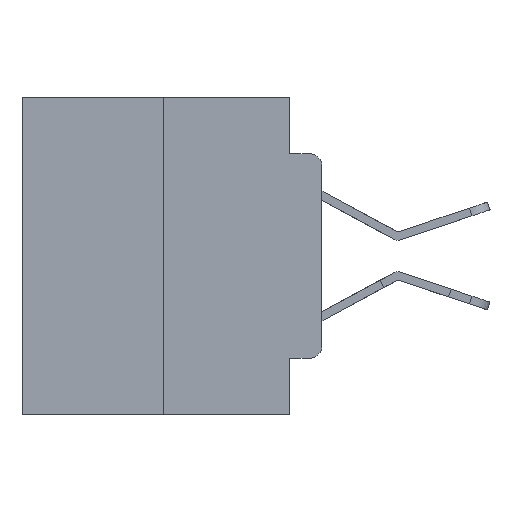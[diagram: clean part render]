
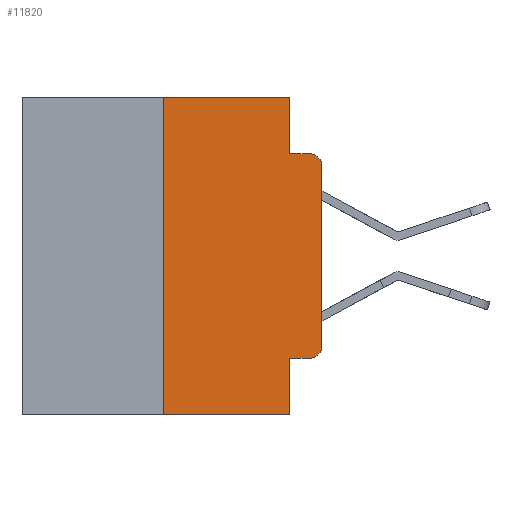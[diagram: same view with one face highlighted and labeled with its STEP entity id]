
A CAD part, left-side view. The second image highlights one B-rep face of the part: STEP entity #11820.
In plain terms, the highlighted planar face has unit normal (-1, 0, 0).
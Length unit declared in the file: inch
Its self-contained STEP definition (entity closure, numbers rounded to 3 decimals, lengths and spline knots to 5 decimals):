
#411 = VERTEX_POINT ( 'NONE', #9035 ) ;
#783 = DIRECTION ( 'NONE',  ( -1., 0., 0. ) ) ;
#877 = LINE ( 'NONE', #20728, #24834 ) ;
#1032 = CARTESIAN_POINT ( 'NONE',  ( 0., 0.051, 0. ) ) ;
#1569 = DIRECTION ( 'NONE',  ( 0., -1., 0. ) ) ;
#1731 = VECTOR ( 'NONE', #1569, 39.37008 ) ;
#1779 = CARTESIAN_POINT ( 'NONE',  ( 0., 0.02, -0.4115 ) ) ;
#2026 = DIRECTION ( 'NONE',  ( 0., 0., 1. ) ) ;
#2052 = CARTESIAN_POINT ( 'NONE',  ( 0., 0.051, -0.4115 ) ) ;
#2334 = ORIENTED_EDGE ( 'NONE', *, *, #18031, .F. ) ;
#2926 = CIRCLE ( 'NONE', #24496, 0.02 ) ;
#3734 = VERTEX_POINT ( 'NONE', #26038 ) ;
#3982 = LINE ( 'NONE', #27919, #9114 ) ;
#4568 = ORIENTED_EDGE ( 'NONE', *, *, #15825, .T. ) ;
#5071 = VERTEX_POINT ( 'NONE', #19744 ) ;
#5751 = EDGE_CURVE ( 'NONE', #28346, #7387, #28324, .T. ) ;
#6058 = VECTOR ( 'NONE', #23178, 39.37008 ) ;
#6081 = ORIENTED_EDGE ( 'NONE', *, *, #9667, .F. ) ;
#6332 = DIRECTION ( 'NONE',  ( 0., -1., 0. ) ) ;
#6353 = ORIENTED_EDGE ( 'NONE', *, *, #12056, .T. ) ;
#6486 = CIRCLE ( 'NONE', #24927, 0.02 ) ;
#7026 = CARTESIAN_POINT ( 'NONE',  ( 0., 0.051, -0.5 ) ) ;
#7074 = ORIENTED_EDGE ( 'NONE', *, *, #5751, .F. ) ;
#7387 = VERTEX_POINT ( 'NONE', #7026 ) ;
#8129 = CARTESIAN_POINT ( 'NONE',  ( 0., 0.473, -0.5 ) ) ;
#8722 = DIRECTION ( 'NONE',  ( 0., 0., -1. ) ) ;
#9000 = CARTESIAN_POINT ( 'NONE',  ( 0., 0.473, 0. ) ) ;
#9035 = CARTESIAN_POINT ( 'NONE',  ( 0., 0., -0.1085 ) ) ;
#9114 = VECTOR ( 'NONE', #23431, 39.37008 ) ;
#9667 = EDGE_CURVE ( 'NONE', #3734, #10769, #22578, .T. ) ;
#9750 = VECTOR ( 'NONE', #2026, 39.37008 ) ;
#9753 = DIRECTION ( 'NONE',  ( 0., 0., -1. ) ) ;
#10661 = VERTEX_POINT ( 'NONE', #22437 ) ;
#10769 = VERTEX_POINT ( 'NONE', #1032 ) ;
#10814 = EDGE_LOOP ( 'NONE', ( #21355, #6353, #24019, #19960, #6081, #2334, #15198, #7074, #4568, #22600 ) ) ;
#11805 = LINE ( 'NONE', #27632, #17343 ) ;
#11819 = DIRECTION ( 'NONE',  ( 0., -1., 0. ) ) ;
#11820 = ADVANCED_FACE ( 'NONE', ( #19510 ), #26118, .F. ) ;
#12056 = EDGE_CURVE ( 'NONE', #411, #10661, #6486, .T. ) ;
#13292 = CARTESIAN_POINT ( 'NONE',  ( 0., 0., 0. ) ) ;
#14021 = CARTESIAN_POINT ( 'NONE',  ( 0., 0.02, -0.3915 ) ) ;
#14335 = VERTEX_POINT ( 'NONE', #1779 ) ;
#14492 = CARTESIAN_POINT ( 'NONE',  ( 0., 0.473, 0. ) ) ;
#14833 = DIRECTION ( 'NONE',  ( 0., -1., 0. ) ) ;
#15198 = ORIENTED_EDGE ( 'NONE', *, *, #21528, .T. ) ;
#15437 = CARTESIAN_POINT ( 'NONE',  ( 0., 0.25, -0.5 ) ) ;
#15595 = LINE ( 'NONE', #13292, #9750 ) ;
#15825 = EDGE_CURVE ( 'NONE', #28346, #14335, #22029, .T. ) ;
#16137 = DIRECTION ( 'NONE',  ( 0., 0., -1. ) ) ;
#16359 = CARTESIAN_POINT ( 'NONE',  ( 0., 0., -0.3915 ) ) ;
#16825 = EDGE_CURVE ( 'NONE', #5071, #10661, #877, .T. ) ;
#17312 = EDGE_CURVE ( 'NONE', #14335, #26269, #2926, .T. ) ;
#17343 = VECTOR ( 'NONE', #23234, 39.37008 ) ;
#17784 = VECTOR ( 'NONE', #14833, 39.37008 ) ;
#18031 = EDGE_CURVE ( 'NONE', #21060, #3734, #11805, .T. ) ;
#18403 = EDGE_CURVE ( 'NONE', #26269, #411, #15595, .T. ) ;
#19510 = FACE_OUTER_BOUND ( 'NONE', #10814, .T. ) ;
#19744 = CARTESIAN_POINT ( 'NONE',  ( 0., 0.051, -0.0885 ) ) ;
#19960 = ORIENTED_EDGE ( 'NONE', *, *, #23476, .F. ) ;
#20005 = AXIS2_PLACEMENT_3D ( 'NONE', #9000, #21820, #8722 ) ;
#20728 = CARTESIAN_POINT ( 'NONE',  ( 0., 0.051, -0.0885 ) ) ;
#21060 = VERTEX_POINT ( 'NONE', #15437 ) ;
#21355 = ORIENTED_EDGE ( 'NONE', *, *, #18403, .T. ) ;
#21528 = EDGE_CURVE ( 'NONE', #21060, #7387, #24926, .T. ) ;
#21820 = DIRECTION ( 'NONE',  ( 1., 0., 0. ) ) ;
#22029 = LINE ( 'NONE', #2052, #25787 ) ;
#22437 = CARTESIAN_POINT ( 'NONE',  ( 0., 0.02, -0.0885 ) ) ;
#22578 = LINE ( 'NONE', #14492, #1731 ) ;
#22600 = ORIENTED_EDGE ( 'NONE', *, *, #17312, .T. ) ;
#23178 = DIRECTION ( 'NONE',  ( 0., 0., -1. ) ) ;
#23234 = DIRECTION ( 'NONE',  ( 0., 0., 1. ) ) ;
#23362 = CARTESIAN_POINT ( 'NONE',  ( 0., 0.051, -0.4115 ) ) ;
#23431 = DIRECTION ( 'NONE',  ( 0., 0., -1. ) ) ;
#23469 = CARTESIAN_POINT ( 'NONE',  ( 0., 0.051, 0. ) ) ;
#23476 = EDGE_CURVE ( 'NONE', #10769, #5071, #3982, .T. ) ;
#24019 = ORIENTED_EDGE ( 'NONE', *, *, #16825, .F. ) ;
#24496 = AXIS2_PLACEMENT_3D ( 'NONE', #14021, #783, #16137 ) ;
#24834 = VECTOR ( 'NONE', #11819, 39.37008 ) ;
#24926 = LINE ( 'NONE', #8129, #17784 ) ;
#24927 = AXIS2_PLACEMENT_3D ( 'NONE', #27354, #27450, #9753 ) ;
#25787 = VECTOR ( 'NONE', #6332, 39.37008 ) ;
#26038 = CARTESIAN_POINT ( 'NONE',  ( 0., 0.25, 0. ) ) ;
#26118 = PLANE ( 'NONE',  #20005 ) ;
#26269 = VERTEX_POINT ( 'NONE', #16359 ) ;
#27354 = CARTESIAN_POINT ( 'NONE',  ( 0., 0.02, -0.1085 ) ) ;
#27450 = DIRECTION ( 'NONE',  ( -1., 0., 0. ) ) ;
#27632 = CARTESIAN_POINT ( 'NONE',  ( 0., 0.25, 0. ) ) ;
#27919 = CARTESIAN_POINT ( 'NONE',  ( 0., 0.051, 0. ) ) ;
#28324 = LINE ( 'NONE', #23469, #6058 ) ;
#28346 = VERTEX_POINT ( 'NONE', #23362 ) ;
